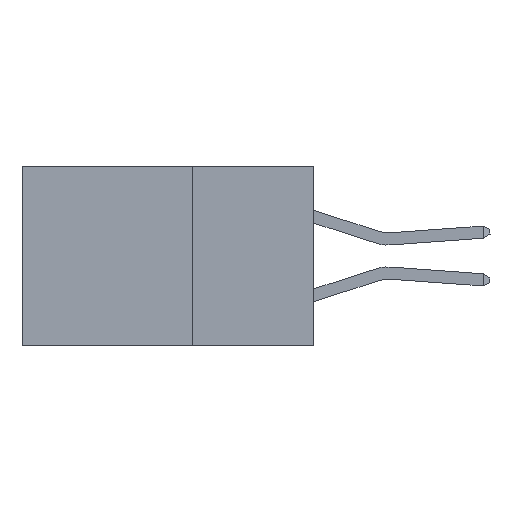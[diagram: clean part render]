
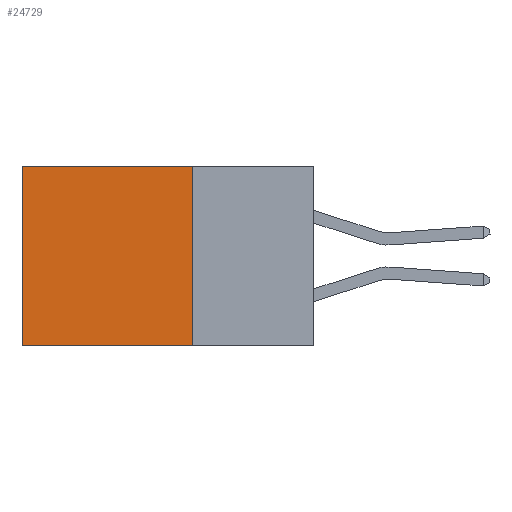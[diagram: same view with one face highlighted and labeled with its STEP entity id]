
A CAD part, left-side view. The second image highlights one B-rep face of the part: STEP entity #24729.
In plain terms, the highlighted planar face has unit normal (-1, 0, 0).
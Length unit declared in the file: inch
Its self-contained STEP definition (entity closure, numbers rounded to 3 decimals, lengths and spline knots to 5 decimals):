
#1879 = VECTOR ( 'NONE', #5773, 39.37008 ) ;
#1880 = EDGE_CURVE ( 'NONE', #24159, #16581, #27069, .T. ) ;
#3523 = DIRECTION ( 'NONE',  ( 1., 0., 0. ) ) ;
#3942 = AXIS2_PLACEMENT_3D ( 'NONE', #27843, #3523, #19099 ) ;
#5773 = DIRECTION ( 'NONE',  ( 0., 1., 0. ) ) ;
#5924 = DIRECTION ( 'NONE',  ( 0., 0., -1. ) ) ;
#5952 = VERTEX_POINT ( 'NONE', #8875 ) ;
#8875 = CARTESIAN_POINT ( 'NONE',  ( 0.2875, 0.6, -0.37 ) ) ;
#8943 = VECTOR ( 'NONE', #25505, 39.37008 ) ;
#9294 = LINE ( 'NONE', #12870, #34525 ) ;
#11951 = CARTESIAN_POINT ( 'NONE',  ( 0.2875, 0.25, 0. ) ) ;
#12870 = CARTESIAN_POINT ( 'NONE',  ( 0.2875, 0.6, 0. ) ) ;
#13372 = CARTESIAN_POINT ( 'NONE',  ( 0.2875, 0.25, -0.37 ) ) ;
#14662 = ORIENTED_EDGE ( 'NONE', *, *, #26471, .T. ) ;
#15299 = CARTESIAN_POINT ( 'NONE',  ( 0.2875, 0.25, 0. ) ) ;
#15491 = LINE ( 'NONE', #15299, #20462 ) ;
#16581 = VERTEX_POINT ( 'NONE', #16886 ) ;
#16886 = CARTESIAN_POINT ( 'NONE',  ( 0.2875, 0.6, 0. ) ) ;
#17434 = EDGE_LOOP ( 'NONE', ( #14662, #19939, #19109, #26663 ) ) ;
#18244 = DIRECTION ( 'NONE',  ( 0., 0., -1. ) ) ;
#19099 = DIRECTION ( 'NONE',  ( 0., 0., -1. ) ) ;
#19109 = ORIENTED_EDGE ( 'NONE', *, *, #21777, .F. ) ;
#19939 = ORIENTED_EDGE ( 'NONE', *, *, #38526, .F. ) ;
#20462 = VECTOR ( 'NONE', #5924, 39.37008 ) ;
#21296 = VERTEX_POINT ( 'NONE', #30086 ) ;
#21777 = EDGE_CURVE ( 'NONE', #24159, #21296, #15491, .T. ) ;
#24159 = VERTEX_POINT ( 'NONE', #39057 ) ;
#24660 = PLANE ( 'NONE',  #3942 ) ;
#24729 = ADVANCED_FACE ( 'NONE', ( #33407 ), #24660, .F. ) ;
#25505 = DIRECTION ( 'NONE',  ( 0., 1., 0. ) ) ;
#26471 = EDGE_CURVE ( 'NONE', #16581, #5952, #9294, .T. ) ;
#26663 = ORIENTED_EDGE ( 'NONE', *, *, #1880, .T. ) ;
#27069 = LINE ( 'NONE', #11951, #1879 ) ;
#27843 = CARTESIAN_POINT ( 'NONE',  ( 0.2875, 0.25, 0. ) ) ;
#30086 = CARTESIAN_POINT ( 'NONE',  ( 0.2875, 0.25, -0.37 ) ) ;
#33407 = FACE_OUTER_BOUND ( 'NONE', #17434, .T. ) ;
#34525 = VECTOR ( 'NONE', #18244, 39.37008 ) ;
#38412 = LINE ( 'NONE', #13372, #8943 ) ;
#38526 = EDGE_CURVE ( 'NONE', #21296, #5952, #38412, .T. ) ;
#39057 = CARTESIAN_POINT ( 'NONE',  ( 0.2875, 0.25, 0. ) ) ;
